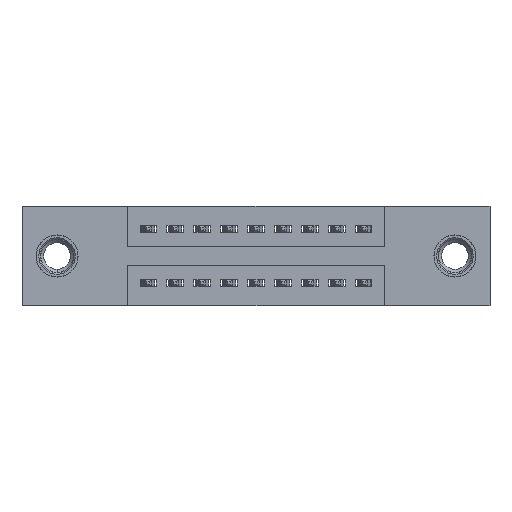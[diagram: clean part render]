
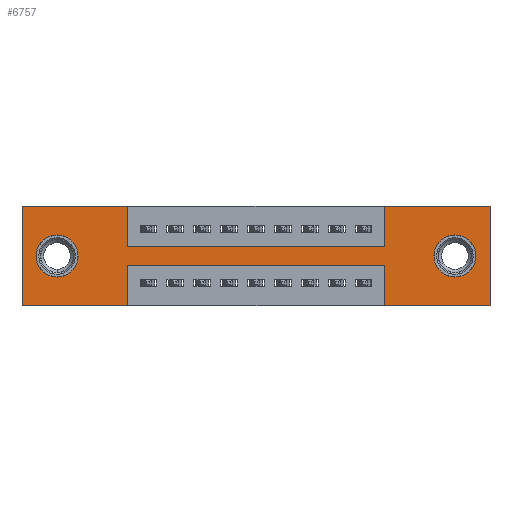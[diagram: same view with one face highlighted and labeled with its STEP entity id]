
A CAD part, front view. The second image highlights one B-rep face of the part: STEP entity #6757.
In plain terms, the highlighted planar face has unit normal (0, -1, 0).
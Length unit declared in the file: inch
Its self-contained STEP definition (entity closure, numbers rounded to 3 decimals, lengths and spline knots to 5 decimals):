
#30 = LINE ( 'NONE', #1870, #9892 ) ;
#374 = LINE ( 'NONE', #11879, #8067 ) ;
#376 = DIRECTION ( 'NONE',  ( 0., 1., 0. ) ) ;
#477 = DIRECTION ( 'NONE',  ( -1., 0., 0. ) ) ;
#717 = EDGE_LOOP ( 'NONE', ( #10392, #11306, #2123, #7627, #10998, #10841, #3439, #7234, #12319, #6795, #1148, #1959 ) ) ;
#788 = LINE ( 'NONE', #6528, #950 ) ;
#821 = EDGE_CURVE ( 'NONE', #7698, #10533, #2801, .T. ) ;
#828 = CARTESIAN_POINT ( 'NONE',  ( 1.605, 0., -0.263 ) ) ;
#950 = VECTOR ( 'NONE', #6648, 39.37008 ) ;
#988 = VECTOR ( 'NONE', #10338, 39.37008 ) ;
#1075 = CARTESIAN_POINT ( 'NONE',  ( 0.3925, 0., -0.15 ) ) ;
#1148 = ORIENTED_EDGE ( 'NONE', *, *, #11497, .F. ) ;
#1307 = EDGE_CURVE ( 'NONE', #12478, #2517, #2495, .T. ) ;
#1393 = VERTEX_POINT ( 'NONE', #5249 ) ;
#1571 = VERTEX_POINT ( 'NONE', #10237 ) ;
#1702 = CARTESIAN_POINT ( 'NONE',  ( 1.3425, 0., 0. ) ) ;
#1713 = VECTOR ( 'NONE', #477, 39.37008 ) ;
#1838 = DIRECTION ( 'NONE',  ( 0., 1., 0. ) ) ;
#1870 = CARTESIAN_POINT ( 'NONE',  ( 1.3425, 0., 0. ) ) ;
#1959 = ORIENTED_EDGE ( 'NONE', *, *, #8978, .F. ) ;
#1961 = EDGE_CURVE ( 'NONE', #5480, #1393, #10608, .T. ) ;
#2123 = ORIENTED_EDGE ( 'NONE', *, *, #7603, .F. ) ;
#2189 = EDGE_CURVE ( 'NONE', #12106, #6069, #2466, .T. ) ;
#2466 = LINE ( 'NONE', #1075, #11679 ) ;
#2495 = LINE ( 'NONE', #11007, #6492 ) ;
#2517 = VERTEX_POINT ( 'NONE', #9303 ) ;
#2636 = DIRECTION ( 'NONE',  ( 0., 0., -1. ) ) ;
#2642 = EDGE_LOOP ( 'NONE', ( #9491, #12111 ) ) ;
#2645 = DIRECTION ( 'NONE',  ( 0., 0., -1. ) ) ;
#2716 = CARTESIAN_POINT ( 'NONE',  ( 0., 0., 0. ) ) ;
#2780 = VERTEX_POINT ( 'NONE', #828 ) ;
#2801 = CIRCLE ( 'NONE', #5421, 0.078 ) ;
#2942 = CARTESIAN_POINT ( 'NONE',  ( 0.3925, 0., -0.22 ) ) ;
#3128 = AXIS2_PLACEMENT_3D ( 'NONE', #7558, #11484, #5586 ) ;
#3301 = CARTESIAN_POINT ( 'NONE',  ( 0.13, 0., -0.185 ) ) ;
#3439 = ORIENTED_EDGE ( 'NONE', *, *, #12613, .F. ) ;
#3583 = CARTESIAN_POINT ( 'NONE',  ( 0., 0., 0. ) ) ;
#3596 = DIRECTION ( 'NONE',  ( 0., 1., 0. ) ) ;
#3721 = DIRECTION ( 'NONE',  ( 1., 0., 0. ) ) ;
#3766 = CARTESIAN_POINT ( 'NONE',  ( 0.3925, 0., 0. ) ) ;
#4019 = AXIS2_PLACEMENT_3D ( 'NONE', #12699, #1838, #4680 ) ;
#4062 = DIRECTION ( 'NONE',  ( 0., 0., 1. ) ) ;
#4108 = EDGE_LOOP ( 'NONE', ( #12580, #4316 ) ) ;
#4126 = CARTESIAN_POINT ( 'NONE',  ( 0.3925, 0., -0.22 ) ) ;
#4316 = ORIENTED_EDGE ( 'NONE', *, *, #12479, .T. ) ;
#4344 = EDGE_CURVE ( 'NONE', #8704, #5480, #7802, .T. ) ;
#4623 = VERTEX_POINT ( 'NONE', #8028 ) ;
#4680 = DIRECTION ( 'NONE',  ( 0., 0., -1. ) ) ;
#4759 = CARTESIAN_POINT ( 'NONE',  ( 0.13, 0., -0.107 ) ) ;
#4800 = AXIS2_PLACEMENT_3D ( 'NONE', #5794, #9702, #9835 ) ;
#4830 = PLANE ( 'NONE',  #4800 ) ;
#5225 = DIRECTION ( 'NONE',  ( 0., 0., 1. ) ) ;
#5249 = CARTESIAN_POINT ( 'NONE',  ( 0.3925, 0., -0.37 ) ) ;
#5368 = LINE ( 'NONE', #9179, #5658 ) ;
#5405 = CIRCLE ( 'NONE', #3128, 0.078 ) ;
#5421 = AXIS2_PLACEMENT_3D ( 'NONE', #3301, #376, #5225 ) ;
#5480 = VERTEX_POINT ( 'NONE', #4126 ) ;
#5544 = LINE ( 'NONE', #6356, #1713 ) ;
#5586 = DIRECTION ( 'NONE',  ( 0., 0., 1. ) ) ;
#5658 = VECTOR ( 'NONE', #7174, 39.37008 ) ;
#5716 = FACE_OUTER_BOUND ( 'NONE', #717, .T. ) ;
#5763 = EDGE_CURVE ( 'NONE', #2780, #12128, #7019, .T. ) ;
#5785 = CIRCLE ( 'NONE', #4019, 0.078 ) ;
#5794 = CARTESIAN_POINT ( 'NONE',  ( 0., 0., -0.37 ) ) ;
#6001 = DIRECTION ( 'NONE',  ( 1., 0., 0. ) ) ;
#6069 = VERTEX_POINT ( 'NONE', #12718 ) ;
#6154 = CARTESIAN_POINT ( 'NONE',  ( 1.735, 0., 0. ) ) ;
#6192 = AXIS2_PLACEMENT_3D ( 'NONE', #9509, #3596, #2645 ) ;
#6356 = CARTESIAN_POINT ( 'NONE',  ( 0., 0., -0.37 ) ) ;
#6492 = VECTOR ( 'NONE', #11053, 39.37008 ) ;
#6528 = CARTESIAN_POINT ( 'NONE',  ( 1.3425, 0., -0.37 ) ) ;
#6534 = EDGE_CURVE ( 'NONE', #6618, #12277, #10982, .T. ) ;
#6618 = VERTEX_POINT ( 'NONE', #2716 ) ;
#6635 = DIRECTION ( 'NONE',  ( 0., 0., -1. ) ) ;
#6648 = DIRECTION ( 'NONE',  ( 0., 0., 1. ) ) ;
#6757 = ADVANCED_FACE ( 'NONE', ( #9310, #12641, #5716 ), #4830, .T. ) ;
#6778 = VECTOR ( 'NONE', #2636, 39.37008 ) ;
#6795 = ORIENTED_EDGE ( 'NONE', *, *, #6534, .F. ) ;
#6925 = CARTESIAN_POINT ( 'NONE',  ( 0.3925, 0., 0. ) ) ;
#7019 = CIRCLE ( 'NONE', #6192, 0.078 ) ;
#7174 = DIRECTION ( 'NONE',  ( -1., 0., 0. ) ) ;
#7234 = ORIENTED_EDGE ( 'NONE', *, *, #2189, .F. ) ;
#7360 = VECTOR ( 'NONE', #9852, 39.37008 ) ;
#7366 = VERTEX_POINT ( 'NONE', #9941 ) ;
#7534 = EDGE_CURVE ( 'NONE', #1571, #7366, #5544, .T. ) ;
#7558 = CARTESIAN_POINT ( 'NONE',  ( 0.13, 0., -0.185 ) ) ;
#7603 = EDGE_CURVE ( 'NONE', #7366, #8704, #788, .T. ) ;
#7627 = ORIENTED_EDGE ( 'NONE', *, *, #7534, .F. ) ;
#7698 = VERTEX_POINT ( 'NONE', #4759 ) ;
#7802 = LINE ( 'NONE', #2942, #7360 ) ;
#8028 = CARTESIAN_POINT ( 'NONE',  ( 0., 0., -0.37 ) ) ;
#8067 = VECTOR ( 'NONE', #4062, 39.37008 ) ;
#8525 = LINE ( 'NONE', #3766, #11895 ) ;
#8704 = VERTEX_POINT ( 'NONE', #12302 ) ;
#8752 = DIRECTION ( 'NONE',  ( 0., 0., 1. ) ) ;
#8978 = EDGE_CURVE ( 'NONE', #1393, #4623, #5368, .T. ) ;
#9179 = CARTESIAN_POINT ( 'NONE',  ( 0., 0., -0.37 ) ) ;
#9303 = CARTESIAN_POINT ( 'NONE',  ( 1.735, 0., 0. ) ) ;
#9310 = FACE_BOUND ( 'NONE', #2642, .T. ) ;
#9491 = ORIENTED_EDGE ( 'NONE', *, *, #9604, .T. ) ;
#9509 = CARTESIAN_POINT ( 'NONE',  ( 1.605, 0., -0.185 ) ) ;
#9604 = EDGE_CURVE ( 'NONE', #12128, #2780, #5785, .T. ) ;
#9610 = LINE ( 'NONE', #6154, #988 ) ;
#9702 = DIRECTION ( 'NONE',  ( 0., -1., 0. ) ) ;
#9835 = DIRECTION ( 'NONE',  ( 0., 0., -1. ) ) ;
#9852 = DIRECTION ( 'NONE',  ( -1., 0., 0. ) ) ;
#9892 = VECTOR ( 'NONE', #8752, 39.37008 ) ;
#9941 = CARTESIAN_POINT ( 'NONE',  ( 1.3425, 0., -0.37 ) ) ;
#10077 = VECTOR ( 'NONE', #3721, 39.37008 ) ;
#10237 = CARTESIAN_POINT ( 'NONE',  ( 1.735, 0., -0.37 ) ) ;
#10338 = DIRECTION ( 'NONE',  ( 0., 0., -1. ) ) ;
#10356 = CARTESIAN_POINT ( 'NONE',  ( 1.605, 0., -0.107 ) ) ;
#10392 = ORIENTED_EDGE ( 'NONE', *, *, #1961, .F. ) ;
#10478 = CARTESIAN_POINT ( 'NONE',  ( 0.3925, 0., -0.15 ) ) ;
#10533 = VERTEX_POINT ( 'NONE', #11983 ) ;
#10608 = LINE ( 'NONE', #11653, #6778 ) ;
#10841 = ORIENTED_EDGE ( 'NONE', *, *, #1307, .F. ) ;
#10982 = LINE ( 'NONE', #3583, #10077 ) ;
#10998 = ORIENTED_EDGE ( 'NONE', *, *, #11601, .F. ) ;
#11007 = CARTESIAN_POINT ( 'NONE',  ( 0., 0., 0. ) ) ;
#11053 = DIRECTION ( 'NONE',  ( 1., 0., 0. ) ) ;
#11306 = ORIENTED_EDGE ( 'NONE', *, *, #4344, .F. ) ;
#11420 = EDGE_CURVE ( 'NONE', #12277, #12106, #8525, .T. ) ;
#11484 = DIRECTION ( 'NONE',  ( 0., 1., 0. ) ) ;
#11497 = EDGE_CURVE ( 'NONE', #4623, #6618, #374, .T. ) ;
#11601 = EDGE_CURVE ( 'NONE', #2517, #1571, #9610, .T. ) ;
#11653 = CARTESIAN_POINT ( 'NONE',  ( 0.3925, 0., -0.37 ) ) ;
#11679 = VECTOR ( 'NONE', #6001, 39.37008 ) ;
#11879 = CARTESIAN_POINT ( 'NONE',  ( 0., 0., 0. ) ) ;
#11895 = VECTOR ( 'NONE', #6635, 39.37008 ) ;
#11983 = CARTESIAN_POINT ( 'NONE',  ( 0.13, 0., -0.263 ) ) ;
#12106 = VERTEX_POINT ( 'NONE', #10478 ) ;
#12111 = ORIENTED_EDGE ( 'NONE', *, *, #5763, .T. ) ;
#12128 = VERTEX_POINT ( 'NONE', #10356 ) ;
#12277 = VERTEX_POINT ( 'NONE', #6925 ) ;
#12302 = CARTESIAN_POINT ( 'NONE',  ( 1.3425, 0., -0.22 ) ) ;
#12319 = ORIENTED_EDGE ( 'NONE', *, *, #11420, .F. ) ;
#12478 = VERTEX_POINT ( 'NONE', #1702 ) ;
#12479 = EDGE_CURVE ( 'NONE', #10533, #7698, #5405, .T. ) ;
#12580 = ORIENTED_EDGE ( 'NONE', *, *, #821, .T. ) ;
#12613 = EDGE_CURVE ( 'NONE', #6069, #12478, #30, .T. ) ;
#12641 = FACE_BOUND ( 'NONE', #4108, .T. ) ;
#12699 = CARTESIAN_POINT ( 'NONE',  ( 1.605, 0., -0.185 ) ) ;
#12718 = CARTESIAN_POINT ( 'NONE',  ( 1.3425, 0., -0.15 ) ) ;
